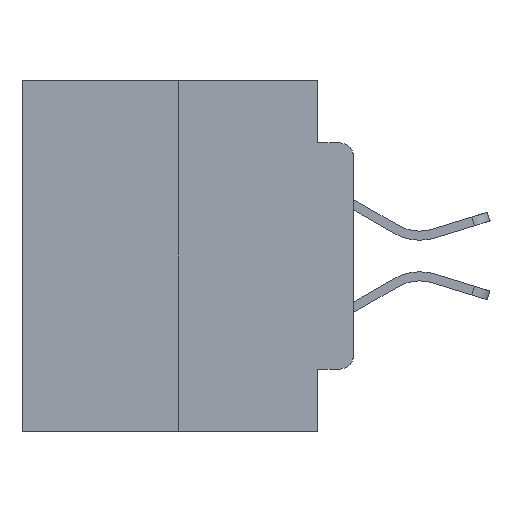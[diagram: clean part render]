
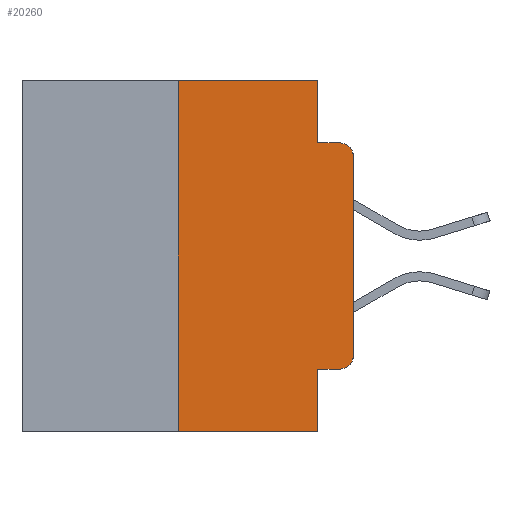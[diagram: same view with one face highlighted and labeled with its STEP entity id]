
A CAD part, left-side view. The second image highlights one B-rep face of the part: STEP entity #20260.
In plain terms, the highlighted planar face has unit normal (-1, 0, 0).
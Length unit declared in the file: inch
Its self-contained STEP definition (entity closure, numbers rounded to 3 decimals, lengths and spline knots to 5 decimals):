
#53 = VECTOR ( 'NONE', #20592, 39.37008 ) ;
#213 = VECTOR ( 'NONE', #5438, 39.37008 ) ;
#410 = CARTESIAN_POINT ( 'NONE',  ( 0., 0.051, -0.5 ) ) ;
#1144 = ORIENTED_EDGE ( 'NONE', *, *, #16914, .T. ) ;
#1160 = CARTESIAN_POINT ( 'NONE',  ( 0., 0.051, 0. ) ) ;
#1276 = DIRECTION ( 'NONE',  ( 0., -1., 0. ) ) ;
#2245 = CARTESIAN_POINT ( 'NONE',  ( 0., 0., -0.1085 ) ) ;
#2374 = DIRECTION ( 'NONE',  ( -1., 0., 0. ) ) ;
#3217 = VERTEX_POINT ( 'NONE', #11364 ) ;
#3238 = CARTESIAN_POINT ( 'NONE',  ( 0., 0.473, -0.5 ) ) ;
#3433 = EDGE_CURVE ( 'NONE', #12104, #4368, #21787, .T. ) ;
#3566 = CARTESIAN_POINT ( 'NONE',  ( 0., 0.473, 0. ) ) ;
#3747 = CARTESIAN_POINT ( 'NONE',  ( 0., 0.051, -0.0885 ) ) ;
#4170 = EDGE_CURVE ( 'NONE', #19887, #25131, #24812, .T. ) ;
#4368 = VERTEX_POINT ( 'NONE', #23387 ) ;
#5438 = DIRECTION ( 'NONE',  ( 0., 0., -1. ) ) ;
#5443 = LINE ( 'NONE', #19983, #15771 ) ;
#5536 = AXIS2_PLACEMENT_3D ( 'NONE', #11735, #25666, #13776 ) ;
#5862 = DIRECTION ( 'NONE',  ( 0., -1., 0. ) ) ;
#6387 = LINE ( 'NONE', #1160, #213 ) ;
#7652 = VERTEX_POINT ( 'NONE', #23363 ) ;
#7864 = VECTOR ( 'NONE', #19340, 39.37008 ) ;
#8234 = EDGE_CURVE ( 'NONE', #7652, #23408, #14620, .T. ) ;
#8360 = ORIENTED_EDGE ( 'NONE', *, *, #4170, .T. ) ;
#8418 = CARTESIAN_POINT ( 'NONE',  ( 0., 0.473, 0. ) ) ;
#8911 = LINE ( 'NONE', #3747, #19001 ) ;
#9456 = VECTOR ( 'NONE', #1276, 39.37008 ) ;
#9957 = DIRECTION ( 'NONE',  ( 0., 0., -1. ) ) ;
#10234 = FACE_OUTER_BOUND ( 'NONE', #20158, .T. ) ;
#10515 = DIRECTION ( 'NONE',  ( 0., -1., 0. ) ) ;
#10983 = ORIENTED_EDGE ( 'NONE', *, *, #3433, .F. ) ;
#11069 = CARTESIAN_POINT ( 'NONE',  ( 0., 0.02, -0.4115 ) ) ;
#11364 = CARTESIAN_POINT ( 'NONE',  ( 0., 0.051, -0.0885 ) ) ;
#11735 = CARTESIAN_POINT ( 'NONE',  ( 0., 0.02, -0.3915 ) ) ;
#12093 = LINE ( 'NONE', #8418, #22702 ) ;
#12104 = VERTEX_POINT ( 'NONE', #25812 ) ;
#12222 = ORIENTED_EDGE ( 'NONE', *, *, #23065, .F. ) ;
#12551 = EDGE_CURVE ( 'NONE', #26238, #19887, #20011, .T. ) ;
#13087 = VERTEX_POINT ( 'NONE', #410 ) ;
#13690 = VERTEX_POINT ( 'NONE', #14684 ) ;
#13776 = DIRECTION ( 'NONE',  ( 0., 0., -1. ) ) ;
#14243 = CARTESIAN_POINT ( 'NONE',  ( 0., 0., -0.3915 ) ) ;
#14453 = ORIENTED_EDGE ( 'NONE', *, *, #24240, .F. ) ;
#14620 = LINE ( 'NONE', #17333, #7864 ) ;
#14684 = CARTESIAN_POINT ( 'NONE',  ( 0., 0.051, 0. ) ) ;
#14813 = CARTESIAN_POINT ( 'NONE',  ( 0., 0.02, -0.1085 ) ) ;
#15086 = ORIENTED_EDGE ( 'NONE', *, *, #17587, .F. ) ;
#15414 = CARTESIAN_POINT ( 'NONE',  ( 0., 0., 0. ) ) ;
#15771 = VECTOR ( 'NONE', #21986, 39.37008 ) ;
#16795 = DIRECTION ( 'NONE',  ( 0., 0., -1. ) ) ;
#16914 = EDGE_CURVE ( 'NONE', #12104, #13087, #25401, .T. ) ;
#17333 = CARTESIAN_POINT ( 'NONE',  ( 0., 0.051, -0.4115 ) ) ;
#17369 = DIRECTION ( 'NONE',  ( 0., 0., 1. ) ) ;
#17587 = EDGE_CURVE ( 'NONE', #13690, #3217, #6387, .T. ) ;
#18481 = ORIENTED_EDGE ( 'NONE', *, *, #12551, .T. ) ;
#18792 = AXIS2_PLACEMENT_3D ( 'NONE', #3566, #21945, #9957 ) ;
#19001 = VECTOR ( 'NONE', #5862, 39.37008 ) ;
#19340 = DIRECTION ( 'NONE',  ( 0., -1., 0. ) ) ;
#19405 = VECTOR ( 'NONE', #17369, 39.37008 ) ;
#19843 = PLANE ( 'NONE',  #18792 ) ;
#19881 = CIRCLE ( 'NONE', #5536, 0.02 ) ;
#19887 = VERTEX_POINT ( 'NONE', #2245 ) ;
#19983 = CARTESIAN_POINT ( 'NONE',  ( 0., 0.051, 0. ) ) ;
#20011 = LINE ( 'NONE', #15414, #19405 ) ;
#20039 = ORIENTED_EDGE ( 'NONE', *, *, #24879, .T. ) ;
#20158 = EDGE_LOOP ( 'NONE', ( #18481, #8360, #14453, #15086, #20969, #10983, #1144, #12222, #24080, #20039 ) ) ;
#20260 = ADVANCED_FACE ( 'NONE', ( #10234 ), #19843, .F. ) ;
#20592 = DIRECTION ( 'NONE',  ( 0., 0., 1. ) ) ;
#20969 = ORIENTED_EDGE ( 'NONE', *, *, #24544, .F. ) ;
#21657 = AXIS2_PLACEMENT_3D ( 'NONE', #14813, #2374, #16795 ) ;
#21787 = LINE ( 'NONE', #22767, #53 ) ;
#21945 = DIRECTION ( 'NONE',  ( 1., 0., 0. ) ) ;
#21986 = DIRECTION ( 'NONE',  ( 0., 0., -1. ) ) ;
#22702 = VECTOR ( 'NONE', #10515, 39.37008 ) ;
#22767 = CARTESIAN_POINT ( 'NONE',  ( 0., 0.25, 0. ) ) ;
#23065 = EDGE_CURVE ( 'NONE', #7652, #13087, #5443, .T. ) ;
#23363 = CARTESIAN_POINT ( 'NONE',  ( 0., 0.051, -0.4115 ) ) ;
#23387 = CARTESIAN_POINT ( 'NONE',  ( 0., 0.25, 0. ) ) ;
#23408 = VERTEX_POINT ( 'NONE', #11069 ) ;
#24080 = ORIENTED_EDGE ( 'NONE', *, *, #8234, .T. ) ;
#24240 = EDGE_CURVE ( 'NONE', #3217, #25131, #8911, .T. ) ;
#24373 = CARTESIAN_POINT ( 'NONE',  ( 0., 0.02, -0.0885 ) ) ;
#24544 = EDGE_CURVE ( 'NONE', #4368, #13690, #12093, .T. ) ;
#24812 = CIRCLE ( 'NONE', #21657, 0.02 ) ;
#24879 = EDGE_CURVE ( 'NONE', #23408, #26238, #19881, .T. ) ;
#25131 = VERTEX_POINT ( 'NONE', #24373 ) ;
#25401 = LINE ( 'NONE', #3238, #9456 ) ;
#25666 = DIRECTION ( 'NONE',  ( -1., 0., 0. ) ) ;
#25812 = CARTESIAN_POINT ( 'NONE',  ( 0., 0.25, -0.5 ) ) ;
#26238 = VERTEX_POINT ( 'NONE', #14243 ) ;
